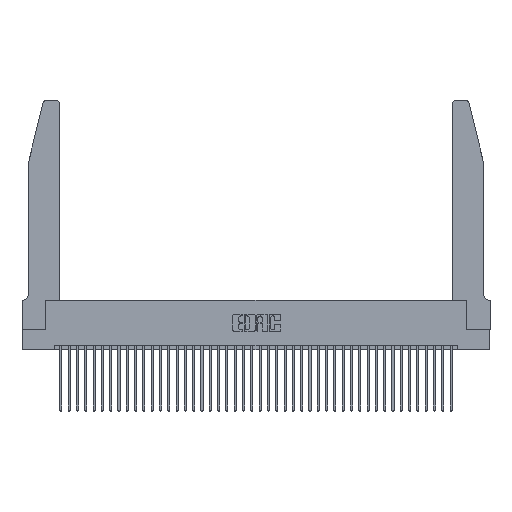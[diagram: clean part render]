
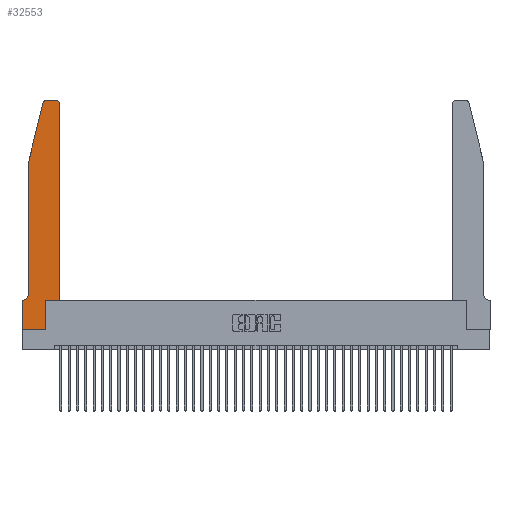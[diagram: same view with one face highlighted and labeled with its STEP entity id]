
A CAD part, top view. The second image highlights one B-rep face of the part: STEP entity #32553.
In plain terms, the highlighted planar face has unit normal (0, 0, 1).
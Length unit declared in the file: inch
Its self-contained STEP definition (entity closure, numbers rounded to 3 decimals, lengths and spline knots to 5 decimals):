
#36 = ORIENTED_EDGE ( 'NONE', *, *, #11216, .T. ) ;
#131 = CIRCLE ( 'NONE', #24064, 0.03 ) ;
#507 = ORIENTED_EDGE ( 'NONE', *, *, #22585, .T. ) ;
#518 = EDGE_CURVE ( 'NONE', #18010, #23240, #25418, .T. ) ;
#1146 = VERTEX_POINT ( 'NONE', #14212 ) ;
#1577 = CARTESIAN_POINT ( 'NONE',  ( 0.0755, 2., 0.37 ) ) ;
#2625 = CARTESIAN_POINT ( 'NONE',  ( 0.0755, 2., 0.37 ) ) ;
#3024 = DIRECTION ( 'NONE',  ( 0., 1., 0. ) ) ;
#3399 = VERTEX_POINT ( 'NONE', #1577 ) ;
#3402 = EDGE_CURVE ( 'NONE', #35904, #5105, #9585, .T. ) ;
#4039 = CARTESIAN_POINT ( 'NONE',  ( 0.0055, 0.42, 0.37 ) ) ;
#4692 = VERTEX_POINT ( 'NONE', #28746 ) ;
#5105 = VERTEX_POINT ( 'NONE', #12453 ) ;
#6375 = CARTESIAN_POINT ( 'NONE',  ( 0.4505, 0.35, 0.37 ) ) ;
#6686 = VERTEX_POINT ( 'NONE', #24741 ) ;
#6800 = EDGE_CURVE ( 'NONE', #3399, #6919, #25717, .T. ) ;
#6919 = VERTEX_POINT ( 'NONE', #18823 ) ;
#7122 = EDGE_LOOP ( 'NONE', ( #18561, #14258, #507, #12764, #36, #20211, #19917, #11527, #32668, #26985, #35333, #21841 ) ) ;
#7464 = VECTOR ( 'NONE', #35817, 39.37008 ) ;
#7571 = VECTOR ( 'NONE', #16553, 39.37008 ) ;
#7876 = DIRECTION ( 'NONE',  ( -1., 0., 0. ) ) ;
#8169 = LINE ( 'NONE', #19669, #10693 ) ;
#8301 = VECTOR ( 'NONE', #20083, 39.37008 ) ;
#8908 = CARTESIAN_POINT ( 'NONE',  ( 0.2865, 0., 0.37 ) ) ;
#9381 = DIRECTION ( 'NONE',  ( -1., 0., 0. ) ) ;
#9585 = CIRCLE ( 'NONE', #15464, 0.03 ) ;
#10410 = EDGE_CURVE ( 'NONE', #19135, #35904, #23457, .T. ) ;
#10693 = VECTOR ( 'NONE', #13058, 39.37008 ) ;
#11216 = EDGE_CURVE ( 'NONE', #6919, #6686, #41520, .T. ) ;
#11527 = ORIENTED_EDGE ( 'NONE', *, *, #28982, .T. ) ;
#11839 = CARTESIAN_POINT ( 'NONE',  ( 0.2865, 0.35, 0.37 ) ) ;
#12393 = EDGE_CURVE ( 'NONE', #34771, #19135, #131, .T. ) ;
#12453 = CARTESIAN_POINT ( 'NONE',  ( 0.25487, 2.72718, 0.37 ) ) ;
#12607 = CARTESIAN_POINT ( 'NONE',  ( 0.4505, 0.35, 0.37 ) ) ;
#12634 = VECTOR ( 'NONE', #16807, 39.37008 ) ;
#12764 = ORIENTED_EDGE ( 'NONE', *, *, #6800, .T. ) ;
#13058 = DIRECTION ( 'NONE',  ( 1., 0., 0. ) ) ;
#13657 = CARTESIAN_POINT ( 'NONE',  ( 0.2605, 2.75, 0.37 ) ) ;
#13879 = DIRECTION ( 'NONE',  ( 0., 0., 1. ) ) ;
#14086 = VECTOR ( 'NONE', #9381, 39.37008 ) ;
#14089 = LINE ( 'NONE', #40818, #32209 ) ;
#14212 = CARTESIAN_POINT ( 'NONE',  ( 0., 0.35, 0.37 ) ) ;
#14258 = ORIENTED_EDGE ( 'NONE', *, *, #3402, .T. ) ;
#15464 = AXIS2_PLACEMENT_3D ( 'NONE', #25194, #40978, #31397 ) ;
#16110 = LINE ( 'NONE', #38781, #14086 ) ;
#16277 = EDGE_CURVE ( 'NONE', #1146, #4692, #14089, .T. ) ;
#16553 = DIRECTION ( 'NONE',  ( 0., -1., 0. ) ) ;
#16645 = VECTOR ( 'NONE', #3024, 39.37008 ) ;
#16807 = DIRECTION ( 'NONE',  ( 0., 1., 0. ) ) ;
#16846 = CARTESIAN_POINT ( 'NONE',  ( 0.4505, 0.35, 0.37 ) ) ;
#17168 = DIRECTION ( 'NONE',  ( -1., 0., 0. ) ) ;
#18010 = VERTEX_POINT ( 'NONE', #11839 ) ;
#18561 = ORIENTED_EDGE ( 'NONE', *, *, #10410, .T. ) ;
#18823 = CARTESIAN_POINT ( 'NONE',  ( 0.0755, 0.42, 0.37 ) ) ;
#19010 = CARTESIAN_POINT ( 'NONE',  ( 0., 0.35, 0.37 ) ) ;
#19099 = VERTEX_POINT ( 'NONE', #8908 ) ;
#19135 = VERTEX_POINT ( 'NONE', #40865 ) ;
#19669 = CARTESIAN_POINT ( 'NONE',  ( 0., 0., 0.37 ) ) ;
#19917 = ORIENTED_EDGE ( 'NONE', *, *, #16277, .T. ) ;
#20083 = DIRECTION ( 'NONE',  ( 1., 0., 0. ) ) ;
#20144 = FACE_OUTER_BOUND ( 'NONE', #7122, .T. ) ;
#20158 = LINE ( 'NONE', #12607, #16645 ) ;
#20211 = ORIENTED_EDGE ( 'NONE', *, *, #22378, .T. ) ;
#21443 = EDGE_CURVE ( 'NONE', #19099, #18010, #40821, .T. ) ;
#21841 = ORIENTED_EDGE ( 'NONE', *, *, #12393, .T. ) ;
#22378 = EDGE_CURVE ( 'NONE', #6686, #1146, #16110, .T. ) ;
#22585 = EDGE_CURVE ( 'NONE', #5105, #3399, #41205, .T. ) ;
#22968 = VECTOR ( 'NONE', #7876, 39.37008 ) ;
#23240 = VERTEX_POINT ( 'NONE', #6375 ) ;
#23457 = LINE ( 'NONE', #13657, #22968 ) ;
#24064 = AXIS2_PLACEMENT_3D ( 'NONE', #39495, #13879, #29909 ) ;
#24741 = CARTESIAN_POINT ( 'NONE',  ( 0.0055, 0.35, 0.37 ) ) ;
#25194 = CARTESIAN_POINT ( 'NONE',  ( 0.284, 2.72, 0.37 ) ) ;
#25418 = LINE ( 'NONE', #16846, #8301 ) ;
#25462 = DIRECTION ( 'NONE',  ( 1., 0., 0. ) ) ;
#25717 = LINE ( 'NONE', #2625, #7571 ) ;
#26482 = CARTESIAN_POINT ( 'NONE',  ( 0.4505, 2.72, 0.37 ) ) ;
#26985 = ORIENTED_EDGE ( 'NONE', *, *, #518, .T. ) ;
#28001 = DIRECTION ( 'NONE',  ( 0., 0., 1. ) ) ;
#28746 = CARTESIAN_POINT ( 'NONE',  ( 0., 0., 0.37 ) ) ;
#28982 = EDGE_CURVE ( 'NONE', #4692, #19099, #8169, .T. ) ;
#29909 = DIRECTION ( 'NONE',  ( 1., 0., 0. ) ) ;
#29940 = DIRECTION ( 'NONE',  ( 0., 0., -1. ) ) ;
#30813 = AXIS2_PLACEMENT_3D ( 'NONE', #19010, #28001, #25462 ) ;
#31330 = CARTESIAN_POINT ( 'NONE',  ( 0.284, 2.75, 0.37 ) ) ;
#31397 = DIRECTION ( 'NONE',  ( 1., 0., 0. ) ) ;
#31809 = PLANE ( 'NONE',  #30813 ) ;
#32209 = VECTOR ( 'NONE', #37139, 39.37008 ) ;
#32424 = CARTESIAN_POINT ( 'NONE',  ( 0.2865, 0.35, 0.37 ) ) ;
#32553 = ADVANCED_FACE ( 'NONE', ( #20144 ), #31809, .T. ) ;
#32668 = ORIENTED_EDGE ( 'NONE', *, *, #21443, .T. ) ;
#33725 = AXIS2_PLACEMENT_3D ( 'NONE', #4039, #29940, #17168 ) ;
#34771 = VERTEX_POINT ( 'NONE', #26482 ) ;
#35333 = ORIENTED_EDGE ( 'NONE', *, *, #37567, .T. ) ;
#35817 = DIRECTION ( 'NONE',  ( -0.239, -0.971, 0. ) ) ;
#35904 = VERTEX_POINT ( 'NONE', #31330 ) ;
#37139 = DIRECTION ( 'NONE',  ( 0., -1., 0. ) ) ;
#37567 = EDGE_CURVE ( 'NONE', #23240, #34771, #20158, .T. ) ;
#38781 = CARTESIAN_POINT ( 'NONE',  ( 0.0755, 0.35, 0.37 ) ) ;
#39209 = CARTESIAN_POINT ( 'NONE',  ( 0.0755, 2., 0.37 ) ) ;
#39495 = CARTESIAN_POINT ( 'NONE',  ( 0.4205, 2.72, 0.37 ) ) ;
#40818 = CARTESIAN_POINT ( 'NONE',  ( 0., 0., 0.37 ) ) ;
#40821 = LINE ( 'NONE', #32424, #12634 ) ;
#40865 = CARTESIAN_POINT ( 'NONE',  ( 0.4205, 2.75, 0.37 ) ) ;
#40978 = DIRECTION ( 'NONE',  ( 0., 0., 1. ) ) ;
#41205 = LINE ( 'NONE', #39209, #7464 ) ;
#41520 = CIRCLE ( 'NONE', #33725, 0.07 ) ;
